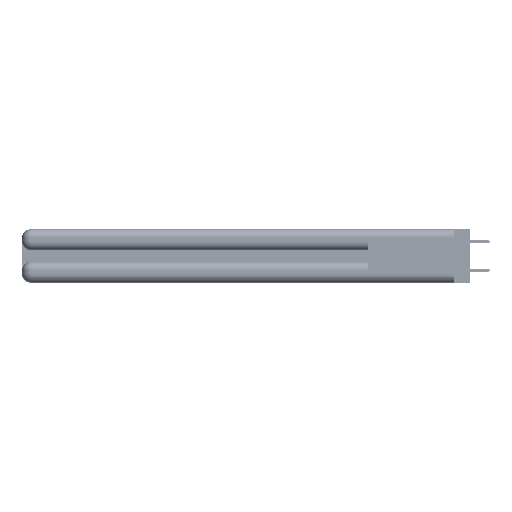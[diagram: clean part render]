
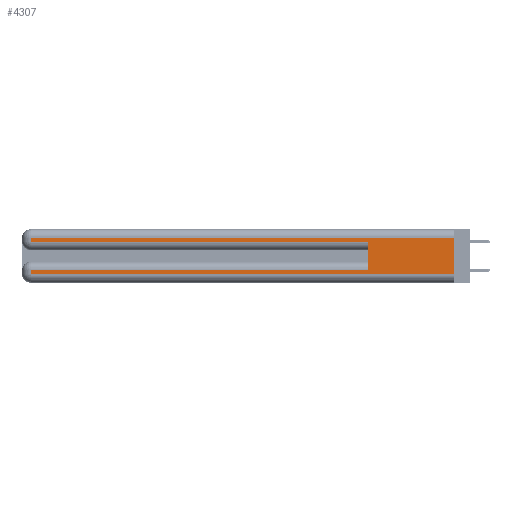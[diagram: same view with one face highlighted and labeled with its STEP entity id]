
A CAD part, left-side view. The second image highlights one B-rep face of the part: STEP entity #4307.
In plain terms, the highlighted planar face has unit normal (-1, 0, 0).
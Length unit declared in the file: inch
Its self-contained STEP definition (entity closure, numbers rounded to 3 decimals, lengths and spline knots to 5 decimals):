
#264 = EDGE_CURVE ( 'NONE', #10865, #32250, #39737, .T. ) ;
#1195 = VERTEX_POINT ( 'NONE', #35577 ) ;
#2775 = CARTESIAN_POINT ( 'NONE',  ( 0., 2.94, 0.31 ) ) ;
#3460 = VERTEX_POINT ( 'NONE', #42034 ) ;
#4024 = AXIS2_PLACEMENT_3D ( 'NONE', #53802, #53983, #27671 ) ;
#4307 = ADVANCED_FACE ( 'NONE', ( #17223 ), #49612, .F. ) ;
#4921 = EDGE_CURVE ( 'NONE', #16698, #45777, #44040, .T. ) ;
#5383 = LINE ( 'NONE', #12117, #18577 ) ;
#6289 = VECTOR ( 'NONE', #51502, 39.37008 ) ;
#6561 = CARTESIAN_POINT ( 'NONE',  ( 0., 0.6, 0.285 ) ) ;
#7371 = CARTESIAN_POINT ( 'NONE',  ( 0., 0.6, 0.145 ) ) ;
#7569 = VERTEX_POINT ( 'NONE', #6561 ) ;
#7948 = DIRECTION ( 'NONE',  ( 0., 0., -1. ) ) ;
#10592 = DIRECTION ( 'NONE',  ( 0., -1., 0. ) ) ;
#10865 = VERTEX_POINT ( 'NONE', #19664 ) ;
#11405 = ORIENTED_EDGE ( 'NONE', *, *, #36661, .T. ) ;
#12117 = CARTESIAN_POINT ( 'NONE',  ( 0., 0., 0.31 ) ) ;
#12284 = LINE ( 'NONE', #37028, #47487 ) ;
#13800 = VECTOR ( 'NONE', #38134, 39.37008 ) ;
#16013 = VECTOR ( 'NONE', #48698, 39.37008 ) ;
#16433 = EDGE_LOOP ( 'NONE', ( #29398, #30282, #11405, #40242, #49303, #50695, #34872, #44292 ) ) ;
#16698 = VERTEX_POINT ( 'NONE', #25867 ) ;
#17223 = FACE_OUTER_BOUND ( 'NONE', #16433, .T. ) ;
#17967 = EDGE_CURVE ( 'NONE', #10865, #7569, #18104, .T. ) ;
#18104 = LINE ( 'NONE', #7371, #6289 ) ;
#18577 = VECTOR ( 'NONE', #42963, 39.37008 ) ;
#19664 = CARTESIAN_POINT ( 'NONE',  ( 0., 0.6, 0.085 ) ) ;
#21341 = CARTESIAN_POINT ( 'NONE',  ( 0., 2.94, 0.37 ) ) ;
#22065 = VERTEX_POINT ( 'NONE', #2775 ) ;
#24838 = CARTESIAN_POINT ( 'NONE',  ( 0., 2.94, 0.37 ) ) ;
#25158 = CARTESIAN_POINT ( 'NONE',  ( 0., 2.94, 0.085 ) ) ;
#25537 = LINE ( 'NONE', #24838, #13800 ) ;
#25867 = CARTESIAN_POINT ( 'NONE',  ( 0., 0., 0.31 ) ) ;
#27671 = DIRECTION ( 'NONE',  ( 0., 0., -1. ) ) ;
#27983 = VECTOR ( 'NONE', #46970, 39.37008 ) ;
#28550 = VECTOR ( 'NONE', #7948, 39.37008 ) ;
#29398 = ORIENTED_EDGE ( 'NONE', *, *, #4921, .F. ) ;
#30282 = ORIENTED_EDGE ( 'NONE', *, *, #56740, .T. ) ;
#31588 = EDGE_CURVE ( 'NONE', #32250, #1195, #25537, .T. ) ;
#32250 = VERTEX_POINT ( 'NONE', #25158 ) ;
#32276 = CARTESIAN_POINT ( 'NONE',  ( 0., 0., 0.37 ) ) ;
#32333 = VECTOR ( 'NONE', #36698, 39.37008 ) ;
#33711 = CARTESIAN_POINT ( 'NONE',  ( 0., 0., 0.085 ) ) ;
#34872 = ORIENTED_EDGE ( 'NONE', *, *, #31588, .T. ) ;
#35577 = CARTESIAN_POINT ( 'NONE',  ( 0., 2.94, 0.06 ) ) ;
#36135 = EDGE_CURVE ( 'NONE', #1195, #45777, #39458, .T. ) ;
#36661 = EDGE_CURVE ( 'NONE', #22065, #3460, #41649, .T. ) ;
#36698 = DIRECTION ( 'NONE',  ( 0., 0., -1. ) ) ;
#37028 = CARTESIAN_POINT ( 'NONE',  ( 0., 0., 0.285 ) ) ;
#38134 = DIRECTION ( 'NONE',  ( 0., 0., -1. ) ) ;
#39458 = LINE ( 'NONE', #44281, #16013 ) ;
#39737 = LINE ( 'NONE', #33711, #27983 ) ;
#40242 = ORIENTED_EDGE ( 'NONE', *, *, #44238, .T. ) ;
#41649 = LINE ( 'NONE', #21341, #28550 ) ;
#42034 = CARTESIAN_POINT ( 'NONE',  ( 0., 2.94, 0.285 ) ) ;
#42963 = DIRECTION ( 'NONE',  ( 0., 1., 0. ) ) ;
#44040 = LINE ( 'NONE', #32276, #32333 ) ;
#44238 = EDGE_CURVE ( 'NONE', #3460, #7569, #12284, .T. ) ;
#44281 = CARTESIAN_POINT ( 'NONE',  ( 0., 0., 0.06 ) ) ;
#44292 = ORIENTED_EDGE ( 'NONE', *, *, #36135, .T. ) ;
#45777 = VERTEX_POINT ( 'NONE', #46491 ) ;
#46491 = CARTESIAN_POINT ( 'NONE',  ( 0., 0., 0.06 ) ) ;
#46970 = DIRECTION ( 'NONE',  ( 0., 1., 0. ) ) ;
#47487 = VECTOR ( 'NONE', #10592, 39.37008 ) ;
#48698 = DIRECTION ( 'NONE',  ( 0., -1., 0. ) ) ;
#49303 = ORIENTED_EDGE ( 'NONE', *, *, #17967, .F. ) ;
#49612 = PLANE ( 'NONE',  #4024 ) ;
#50695 = ORIENTED_EDGE ( 'NONE', *, *, #264, .T. ) ;
#51502 = DIRECTION ( 'NONE',  ( 0., 0., 1. ) ) ;
#53802 = CARTESIAN_POINT ( 'NONE',  ( 0., 0., 0.37 ) ) ;
#53983 = DIRECTION ( 'NONE',  ( 1., 0., 0. ) ) ;
#56740 = EDGE_CURVE ( 'NONE', #16698, #22065, #5383, .T. ) ;
